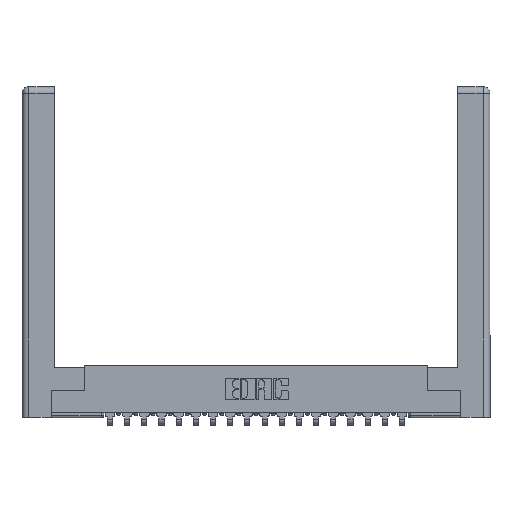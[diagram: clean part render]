
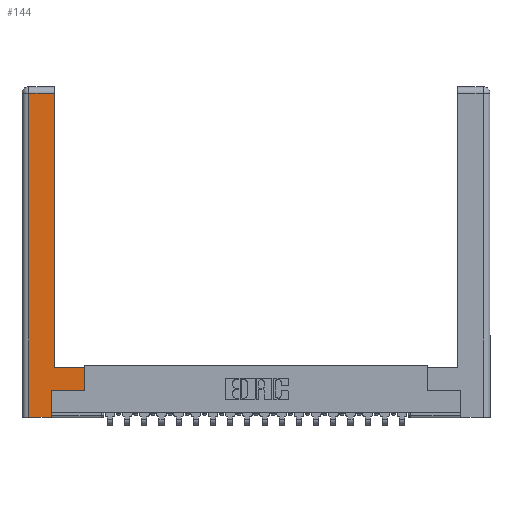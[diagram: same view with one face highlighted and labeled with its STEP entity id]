
A CAD part, top view. The second image highlights one B-rep face of the part: STEP entity #144.
In plain terms, the highlighted planar face has unit normal (0, 0, 1).
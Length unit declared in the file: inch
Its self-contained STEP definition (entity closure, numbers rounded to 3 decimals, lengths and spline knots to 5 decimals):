
#138 = EDGE_CURVE ( 'NONE', #12711, #13557, #14308, .T. ) ;
#144 = ADVANCED_FACE ( 'NONE', ( #1424 ), #17694, .F. ) ;
#890 = EDGE_CURVE ( 'NONE', #6753, #1457, #7190, .T. ) ;
#892 = DIRECTION ( 'NONE',  ( 0., 1., 0. ) ) ;
#1424 = FACE_OUTER_BOUND ( 'NONE', #19044, .T. ) ;
#1457 = VERTEX_POINT ( 'NONE', #19238 ) ;
#1523 = CARTESIAN_POINT ( 'NONE',  ( 0., 0., 0. ) ) ;
#1827 = ORIENTED_EDGE ( 'NONE', *, *, #890, .T. ) ;
#2031 = ORIENTED_EDGE ( 'NONE', *, *, #6274, .T. ) ;
#2123 = VERTEX_POINT ( 'NONE', #12016 ) ;
#2169 = LINE ( 'NONE', #20354, #10271 ) ;
#2315 = CARTESIAN_POINT ( 'NONE',  ( 0.565, 0.245, 0. ) ) ;
#2676 = VECTOR ( 'NONE', #7925, 39.37008 ) ;
#4598 = ORIENTED_EDGE ( 'NONE', *, *, #138, .T. ) ;
#4805 = CARTESIAN_POINT ( 'NONE',  ( 0.265, 0.245, 0. ) ) ;
#4872 = DIRECTION ( 'NONE',  ( 1., 0., 0. ) ) ;
#5288 = CARTESIAN_POINT ( 'NONE',  ( 0.565, 0.45, 0. ) ) ;
#6274 = EDGE_CURVE ( 'NONE', #2123, #10386, #2169, .T. ) ;
#6753 = VERTEX_POINT ( 'NONE', #18066 ) ;
#6905 = ORIENTED_EDGE ( 'NONE', *, *, #14065, .T. ) ;
#7190 = LINE ( 'NONE', #17123, #7335 ) ;
#7335 = VECTOR ( 'NONE', #10726, 39.37008 ) ;
#7925 = DIRECTION ( 'NONE',  ( 1., 0., 0. ) ) ;
#8065 = CARTESIAN_POINT ( 'NONE',  ( 0.295, 2.94, 0. ) ) ;
#8331 = LINE ( 'NONE', #19330, #2676 ) ;
#8455 = DIRECTION ( 'NONE',  ( -1., 0., 0. ) ) ;
#8854 = ORIENTED_EDGE ( 'NONE', *, *, #12839, .T. ) ;
#8856 = DIRECTION ( 'NONE',  ( 0., 1., 0. ) ) ;
#10271 = VECTOR ( 'NONE', #892, 39.37008 ) ;
#10366 = VERTEX_POINT ( 'NONE', #5288 ) ;
#10386 = VERTEX_POINT ( 'NONE', #8065 ) ;
#10726 = DIRECTION ( 'NONE',  ( 0., -1., 0. ) ) ;
#10964 = LINE ( 'NONE', #20767, #13889 ) ;
#11290 = EDGE_CURVE ( 'NONE', #1457, #20245, #8331, .T. ) ;
#11356 = LINE ( 'NONE', #11550, #18728 ) ;
#11550 = CARTESIAN_POINT ( 'NONE',  ( 0.295, 0.45, 0. ) ) ;
#11615 = VECTOR ( 'NONE', #15584, 39.37008 ) ;
#12016 = CARTESIAN_POINT ( 'NONE',  ( 0.295, 0.45, 0. ) ) ;
#12571 = CARTESIAN_POINT ( 'NONE',  ( 0.565, 0.245, 0. ) ) ;
#12711 = VERTEX_POINT ( 'NONE', #4805 ) ;
#12774 = DIRECTION ( 'NONE',  ( -1., 0., 0. ) ) ;
#12839 = EDGE_CURVE ( 'NONE', #13557, #10366, #15269, .T. ) ;
#13557 = VERTEX_POINT ( 'NONE', #2315 ) ;
#13695 = VECTOR ( 'NONE', #4872, 39.37008 ) ;
#13889 = VECTOR ( 'NONE', #12774, 39.37008 ) ;
#14065 = EDGE_CURVE ( 'NONE', #20245, #12711, #16003, .T. ) ;
#14224 = CARTESIAN_POINT ( 'NONE',  ( 0.265, 0.245, 0. ) ) ;
#14308 = LINE ( 'NONE', #12571, #13695 ) ;
#14423 = EDGE_CURVE ( 'NONE', #10386, #6753, #10964, .T. ) ;
#14602 = EDGE_CURVE ( 'NONE', #10366, #2123, #11356, .T. ) ;
#15253 = ORIENTED_EDGE ( 'NONE', *, *, #14423, .T. ) ;
#15269 = LINE ( 'NONE', #16968, #21119 ) ;
#15584 = DIRECTION ( 'NONE',  ( 0., 1., 0. ) ) ;
#15892 = DIRECTION ( 'NONE',  ( -1., 0., 0. ) ) ;
#16003 = LINE ( 'NONE', #14224, #11615 ) ;
#16121 = ORIENTED_EDGE ( 'NONE', *, *, #11290, .T. ) ;
#16238 = CARTESIAN_POINT ( 'NONE',  ( 0.265, 0., 0. ) ) ;
#16968 = CARTESIAN_POINT ( 'NONE',  ( 0.565, 0.45, 0. ) ) ;
#17123 = CARTESIAN_POINT ( 'NONE',  ( 0.0615, 0., 0. ) ) ;
#17324 = ORIENTED_EDGE ( 'NONE', *, *, #14602, .T. ) ;
#17694 = PLANE ( 'NONE',  #19477 ) ;
#18066 = CARTESIAN_POINT ( 'NONE',  ( 0.0615, 2.94, 0. ) ) ;
#18728 = VECTOR ( 'NONE', #8455, 39.37008 ) ;
#19044 = EDGE_LOOP ( 'NONE', ( #2031, #15253, #1827, #16121, #6905, #4598, #8854, #17324 ) ) ;
#19238 = CARTESIAN_POINT ( 'NONE',  ( 0.0615, 0., 0. ) ) ;
#19330 = CARTESIAN_POINT ( 'NONE',  ( 0.265, 0., 0. ) ) ;
#19477 = AXIS2_PLACEMENT_3D ( 'NONE', #1523, #20686, #15892 ) ;
#20245 = VERTEX_POINT ( 'NONE', #16238 ) ;
#20354 = CARTESIAN_POINT ( 'NONE',  ( 0.295, 3., 0. ) ) ;
#20686 = DIRECTION ( 'NONE',  ( 0., 0., -1. ) ) ;
#20767 = CARTESIAN_POINT ( 'NONE',  ( 0.0615, 2.94, 0. ) ) ;
#21119 = VECTOR ( 'NONE', #8856, 39.37008 ) ;
